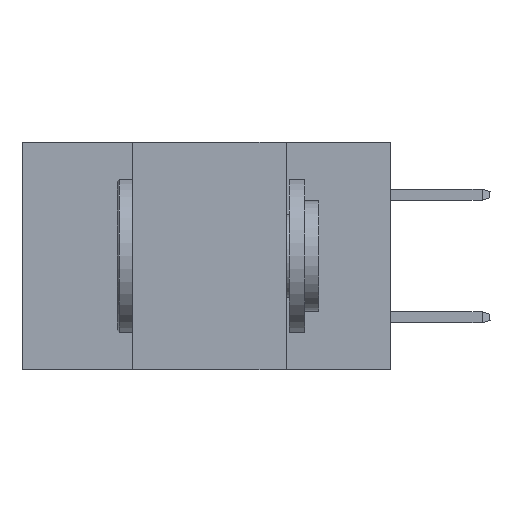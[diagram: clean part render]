
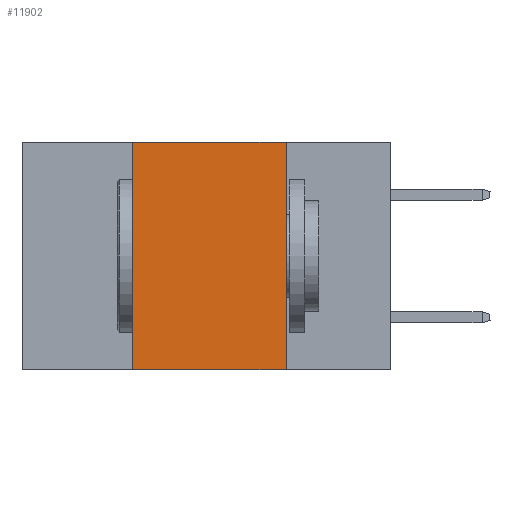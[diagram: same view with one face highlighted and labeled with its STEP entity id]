
A CAD part, left-side view. The second image highlights one B-rep face of the part: STEP entity #11902.
In plain terms, the highlighted planar face has unit normal (-1, 0, 0).
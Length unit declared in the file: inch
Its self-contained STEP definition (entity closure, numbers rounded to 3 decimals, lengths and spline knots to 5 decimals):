
#94 = DIRECTION ( 'NONE',  ( 0., 0., 1. ) ) ;
#154 = CARTESIAN_POINT ( 'NONE',  ( 0., 0.17, -0.37 ) ) ;
#1312 = EDGE_CURVE ( 'NONE', #1600, #12010, #10581, .T. ) ;
#1335 = DIRECTION ( 'NONE',  ( 0., 0., -1. ) ) ;
#1351 = CARTESIAN_POINT ( 'NONE',  ( 0., 0.17, 0. ) ) ;
#1507 = CARTESIAN_POINT ( 'NONE',  ( 0., 0.6, 0. ) ) ;
#1600 = VERTEX_POINT ( 'NONE', #5430 ) ;
#2091 = ORIENTED_EDGE ( 'NONE', *, *, #5809, .F. ) ;
#2289 = VECTOR ( 'NONE', #6012, 39.37008 ) ;
#2492 = LINE ( 'NONE', #1507, #7490 ) ;
#2949 = CARTESIAN_POINT ( 'NONE',  ( 0., 0.42, 0. ) ) ;
#3107 = VECTOR ( 'NONE', #94, 39.37008 ) ;
#3906 = EDGE_CURVE ( 'NONE', #1600, #4933, #12230, .T. ) ;
#4579 = ORIENTED_EDGE ( 'NONE', *, *, #8596, .F. ) ;
#4933 = VERTEX_POINT ( 'NONE', #154 ) ;
#5007 = PLANE ( 'NONE',  #9024 ) ;
#5430 = CARTESIAN_POINT ( 'NONE',  ( 0., 0.42, -0.37 ) ) ;
#5809 = EDGE_CURVE ( 'NONE', #6139, #4933, #10921, .T. ) ;
#5991 = DIRECTION ( 'NONE',  ( 0., 0., -1. ) ) ;
#6012 = DIRECTION ( 'NONE',  ( 0., -1., 0. ) ) ;
#6051 = CARTESIAN_POINT ( 'NONE',  ( 0., 0.6, -0.37 ) ) ;
#6139 = VERTEX_POINT ( 'NONE', #10100 ) ;
#7134 = ORIENTED_EDGE ( 'NONE', *, *, #1312, .F. ) ;
#7257 = DIRECTION ( 'NONE',  ( 0., -1., 0. ) ) ;
#7490 = VECTOR ( 'NONE', #7257, 39.37008 ) ;
#8596 = EDGE_CURVE ( 'NONE', #12010, #6139, #2492, .T. ) ;
#8856 = CARTESIAN_POINT ( 'NONE',  ( 0., 0.42, 0. ) ) ;
#9014 = VECTOR ( 'NONE', #1335, 39.37008 ) ;
#9024 = AXIS2_PLACEMENT_3D ( 'NONE', #10638, #11545, #5991 ) ;
#9961 = EDGE_LOOP ( 'NONE', ( #2091, #4579, #7134, #12063 ) ) ;
#10100 = CARTESIAN_POINT ( 'NONE',  ( 0., 0.17, 0. ) ) ;
#10581 = LINE ( 'NONE', #2949, #3107 ) ;
#10638 = CARTESIAN_POINT ( 'NONE',  ( 0., 0.6, 0. ) ) ;
#10921 = LINE ( 'NONE', #1351, #9014 ) ;
#11375 = FACE_OUTER_BOUND ( 'NONE', #9961, .T. ) ;
#11545 = DIRECTION ( 'NONE',  ( 1., 0., 0. ) ) ;
#11902 = ADVANCED_FACE ( 'NONE', ( #11375 ), #5007, .F. ) ;
#12010 = VERTEX_POINT ( 'NONE', #8856 ) ;
#12063 = ORIENTED_EDGE ( 'NONE', *, *, #3906, .T. ) ;
#12230 = LINE ( 'NONE', #6051, #2289 ) ;
